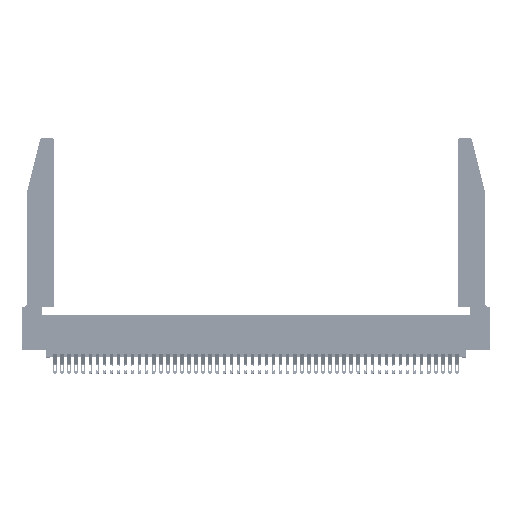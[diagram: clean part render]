
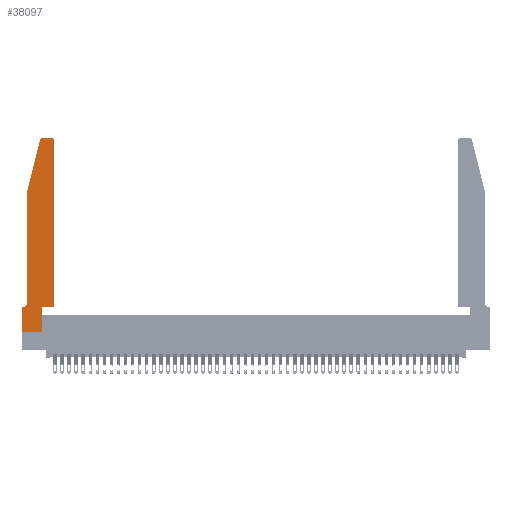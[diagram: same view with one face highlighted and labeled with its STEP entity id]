
A CAD part, top view. The second image highlights one B-rep face of the part: STEP entity #38097.
In plain terms, the highlighted planar face has unit normal (0, 0, 1).
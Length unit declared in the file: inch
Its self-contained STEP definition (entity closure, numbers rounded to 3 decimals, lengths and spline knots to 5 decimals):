
#302 = EDGE_CURVE ( 'NONE', #32954, #16315, #20631, .T. ) ;
#1197 = LINE ( 'NONE', #12772, #26417 ) ;
#1470 = DIRECTION ( 'NONE',  ( 1., 0., 0. ) ) ;
#1689 = CARTESIAN_POINT ( 'NONE',  ( 0.4505, 0.35, 0.37 ) ) ;
#2495 = DIRECTION ( 'NONE',  ( -1., 0., 0. ) ) ;
#2998 = VECTOR ( 'NONE', #21133, 39.37008 ) ;
#3140 = DIRECTION ( 'NONE',  ( 0., 0., -1. ) ) ;
#3170 = CARTESIAN_POINT ( 'NONE',  ( 0., 0.35, 0.37 ) ) ;
#3212 = EDGE_LOOP ( 'NONE', ( #16515, #13050, #35560, #42364, #6786, #5008, #12433, #7182, #33954, #27829, #22730, #40504 ) ) ;
#5008 = ORIENTED_EDGE ( 'NONE', *, *, #302, .T. ) ;
#5902 = VERTEX_POINT ( 'NONE', #26837 ) ;
#6691 = DIRECTION ( 'NONE',  ( -1., 0., 0. ) ) ;
#6756 = EDGE_CURVE ( 'NONE', #41493, #38840, #42642, .T. ) ;
#6786 = ORIENTED_EDGE ( 'NONE', *, *, #16790, .T. ) ;
#7182 = ORIENTED_EDGE ( 'NONE', *, *, #37191, .T. ) ;
#7558 = VECTOR ( 'NONE', #1470, 39.37008 ) ;
#8249 = CARTESIAN_POINT ( 'NONE',  ( 0.0755, 0.42, 0.37 ) ) ;
#8480 = DIRECTION ( 'NONE',  ( -1., 0., 0. ) ) ;
#8740 = CARTESIAN_POINT ( 'NONE',  ( 0., 0., 0.37 ) ) ;
#9077 = CARTESIAN_POINT ( 'NONE',  ( 0., 0., 0.37 ) ) ;
#9785 = CIRCLE ( 'NONE', #35862, 0.03 ) ;
#10511 = LINE ( 'NONE', #9077, #12311 ) ;
#11090 = VERTEX_POINT ( 'NONE', #34499 ) ;
#12311 = VECTOR ( 'NONE', #31576, 39.37008 ) ;
#12433 = ORIENTED_EDGE ( 'NONE', *, *, #13488, .T. ) ;
#12772 = CARTESIAN_POINT ( 'NONE',  ( 0.0755, 2., 0.37 ) ) ;
#13001 = LINE ( 'NONE', #46719, #2998 ) ;
#13050 = ORIENTED_EDGE ( 'NONE', *, *, #17315, .T. ) ;
#13488 = EDGE_CURVE ( 'NONE', #16315, #30246, #10511, .T. ) ;
#13836 = AXIS2_PLACEMENT_3D ( 'NONE', #36448, #21357, #47593 ) ;
#14202 = CARTESIAN_POINT ( 'NONE',  ( 0.284, 2.72, 0.37 ) ) ;
#14942 = VERTEX_POINT ( 'NONE', #35430 ) ;
#15374 = FACE_OUTER_BOUND ( 'NONE', #3212, .T. ) ;
#15642 = DIRECTION ( 'NONE',  ( 0., 0., 1. ) ) ;
#15944 = CARTESIAN_POINT ( 'NONE',  ( 0.0755, 2., 0.37 ) ) ;
#16315 = VERTEX_POINT ( 'NONE', #3170 ) ;
#16515 = ORIENTED_EDGE ( 'NONE', *, *, #21893, .T. ) ;
#16790 = EDGE_CURVE ( 'NONE', #40334, #32954, #23067, .T. ) ;
#16953 = LINE ( 'NONE', #24242, #7558 ) ;
#17315 = EDGE_CURVE ( 'NONE', #41574, #11090, #9785, .T. ) ;
#17878 = CARTESIAN_POINT ( 'NONE',  ( 0.2865, 0., 0.37 ) ) ;
#18118 = CARTESIAN_POINT ( 'NONE',  ( 0.0755, 0.35, 0.37 ) ) ;
#18229 = CARTESIAN_POINT ( 'NONE',  ( 0.0055, 0.35, 0.37 ) ) ;
#19096 = CARTESIAN_POINT ( 'NONE',  ( 0., 0.35, 0.37 ) ) ;
#19416 = PLANE ( 'NONE',  #38721 ) ;
#20196 = EDGE_CURVE ( 'NONE', #5902, #41493, #16953, .T. ) ;
#20631 = LINE ( 'NONE', #18118, #31783 ) ;
#21133 = DIRECTION ( 'NONE',  ( 1., 0., 0. ) ) ;
#21357 = DIRECTION ( 'NONE',  ( 0., 0., 1. ) ) ;
#21893 = EDGE_CURVE ( 'NONE', #37629, #41574, #25623, .T. ) ;
#22309 = VECTOR ( 'NONE', #23677, 39.37008 ) ;
#22730 = ORIENTED_EDGE ( 'NONE', *, *, #6756, .T. ) ;
#23067 = CIRCLE ( 'NONE', #38012, 0.07 ) ;
#23306 = DIRECTION ( 'NONE',  ( 0., 1., 0. ) ) ;
#23677 = DIRECTION ( 'NONE',  ( -0.239, -0.971, 0. ) ) ;
#24242 = CARTESIAN_POINT ( 'NONE',  ( 0.4505, 0.35, 0.37 ) ) ;
#24982 = VECTOR ( 'NONE', #8480, 39.37008 ) ;
#25623 = LINE ( 'NONE', #42150, #24982 ) ;
#25707 = DIRECTION ( 'NONE',  ( 1., 0., 0. ) ) ;
#26417 = VECTOR ( 'NONE', #42961, 39.37008 ) ;
#26837 = CARTESIAN_POINT ( 'NONE',  ( 0.2865, 0.35, 0.37 ) ) ;
#26879 = LINE ( 'NONE', #45638, #31031 ) ;
#27561 = CIRCLE ( 'NONE', #13836, 0.03 ) ;
#27829 = ORIENTED_EDGE ( 'NONE', *, *, #20196, .T. ) ;
#29871 = LINE ( 'NONE', #15944, #22309 ) ;
#30246 = VERTEX_POINT ( 'NONE', #8740 ) ;
#30634 = CARTESIAN_POINT ( 'NONE',  ( 0.4205, 2.75, 0.37 ) ) ;
#30774 = EDGE_CURVE ( 'NONE', #38563, #5902, #26879, .T. ) ;
#31031 = VECTOR ( 'NONE', #41862, 39.37008 ) ;
#31576 = DIRECTION ( 'NONE',  ( 0., -1., 0. ) ) ;
#31783 = VECTOR ( 'NONE', #6691, 39.37008 ) ;
#32954 = VERTEX_POINT ( 'NONE', #18229 ) ;
#33954 = ORIENTED_EDGE ( 'NONE', *, *, #30774, .T. ) ;
#34454 = VECTOR ( 'NONE', #23306, 39.37008 ) ;
#34499 = CARTESIAN_POINT ( 'NONE',  ( 0.25487, 2.72718, 0.37 ) ) ;
#35233 = EDGE_CURVE ( 'NONE', #14942, #40334, #1197, .T. ) ;
#35430 = CARTESIAN_POINT ( 'NONE',  ( 0.0755, 2., 0.37 ) ) ;
#35560 = ORIENTED_EDGE ( 'NONE', *, *, #36294, .T. ) ;
#35636 = CARTESIAN_POINT ( 'NONE',  ( 0.284, 2.75, 0.37 ) ) ;
#35862 = AXIS2_PLACEMENT_3D ( 'NONE', #14202, #40784, #25707 ) ;
#36294 = EDGE_CURVE ( 'NONE', #11090, #14942, #29871, .T. ) ;
#36448 = CARTESIAN_POINT ( 'NONE',  ( 0.4205, 2.72, 0.37 ) ) ;
#36634 = EDGE_CURVE ( 'NONE', #38840, #37629, #27561, .T. ) ;
#37191 = EDGE_CURVE ( 'NONE', #30246, #38563, #13001, .T. ) ;
#37629 = VERTEX_POINT ( 'NONE', #30634 ) ;
#38012 = AXIS2_PLACEMENT_3D ( 'NONE', #47573, #3140, #2495 ) ;
#38097 = ADVANCED_FACE ( 'NONE', ( #15374 ), #19416, .T. ) ;
#38563 = VERTEX_POINT ( 'NONE', #17878 ) ;
#38721 = AXIS2_PLACEMENT_3D ( 'NONE', #19096, #15642, #41929 ) ;
#38840 = VERTEX_POINT ( 'NONE', #42030 ) ;
#40334 = VERTEX_POINT ( 'NONE', #8249 ) ;
#40504 = ORIENTED_EDGE ( 'NONE', *, *, #36634, .T. ) ;
#40784 = DIRECTION ( 'NONE',  ( 0., 0., 1. ) ) ;
#41493 = VERTEX_POINT ( 'NONE', #1689 ) ;
#41574 = VERTEX_POINT ( 'NONE', #35636 ) ;
#41862 = DIRECTION ( 'NONE',  ( 0., 1., 0. ) ) ;
#41929 = DIRECTION ( 'NONE',  ( 1., 0., 0. ) ) ;
#42030 = CARTESIAN_POINT ( 'NONE',  ( 0.4505, 2.72, 0.37 ) ) ;
#42150 = CARTESIAN_POINT ( 'NONE',  ( 0.2605, 2.75, 0.37 ) ) ;
#42364 = ORIENTED_EDGE ( 'NONE', *, *, #35233, .T. ) ;
#42642 = LINE ( 'NONE', #43029, #34454 ) ;
#42961 = DIRECTION ( 'NONE',  ( 0., -1., 0. ) ) ;
#43029 = CARTESIAN_POINT ( 'NONE',  ( 0.4505, 0.35, 0.37 ) ) ;
#45638 = CARTESIAN_POINT ( 'NONE',  ( 0.2865, 0.35, 0.37 ) ) ;
#46719 = CARTESIAN_POINT ( 'NONE',  ( 0., 0., 0.37 ) ) ;
#47573 = CARTESIAN_POINT ( 'NONE',  ( 0.0055, 0.42, 0.37 ) ) ;
#47593 = DIRECTION ( 'NONE',  ( 1., 0., 0. ) ) ;
